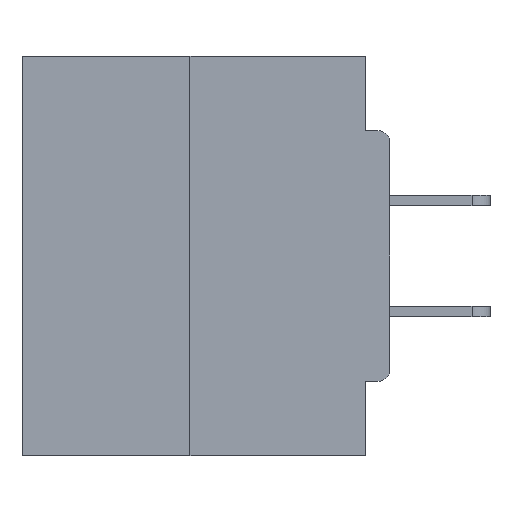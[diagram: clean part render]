
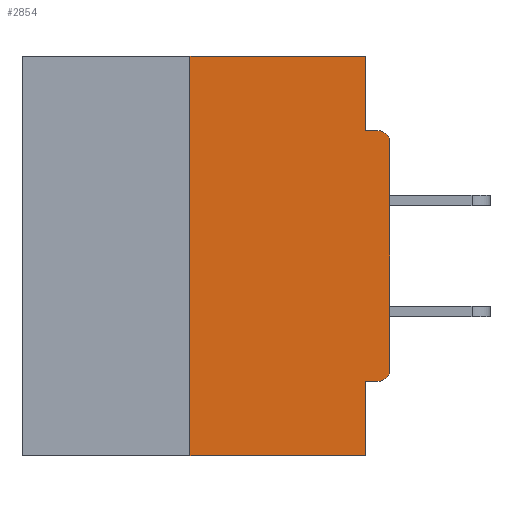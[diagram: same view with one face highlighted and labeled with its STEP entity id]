
A CAD part, left-side view. The second image highlights one B-rep face of the part: STEP entity #2854.
In plain terms, the highlighted planar face has unit normal (-1, 0, 0).
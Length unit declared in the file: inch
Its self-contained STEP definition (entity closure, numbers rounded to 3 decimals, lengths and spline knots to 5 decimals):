
#128 = CARTESIAN_POINT ( 'NONE',  ( 0., 0.25, 0. ) ) ;
#163 = LINE ( 'NONE', #9701, #3685 ) ;
#194 = LINE ( 'NONE', #17991, #10735 ) ;
#793 = EDGE_CURVE ( 'NONE', #3441, #19362, #4950, .T. ) ;
#2200 = VECTOR ( 'NONE', #20018, 39.37008 ) ;
#2360 = CARTESIAN_POINT ( 'NONE',  ( 0., 0.015, -0.0935 ) ) ;
#2854 = ADVANCED_FACE ( 'NONE', ( #17640 ), #22155, .F. ) ;
#3117 = CARTESIAN_POINT ( 'NONE',  ( 0., 0.031, -0.0935 ) ) ;
#3195 = AXIS2_PLACEMENT_3D ( 'NONE', #13177, #10878, #30624 ) ;
#3441 = VERTEX_POINT ( 'NONE', #32235 ) ;
#3685 = VECTOR ( 'NONE', #22270, 39.37008 ) ;
#4775 = LINE ( 'NONE', #26997, #11666 ) ;
#4950 = LINE ( 'NONE', #18474, #13860 ) ;
#4961 = ORIENTED_EDGE ( 'NONE', *, *, #5586, .T. ) ;
#5586 = EDGE_CURVE ( 'NONE', #31996, #8220, #15919, .T. ) ;
#6318 = VERTEX_POINT ( 'NONE', #6709 ) ;
#6709 = CARTESIAN_POINT ( 'NONE',  ( 0., 0.031, -0.4065 ) ) ;
#7233 = VECTOR ( 'NONE', #26794, 39.37008 ) ;
#7288 = VERTEX_POINT ( 'NONE', #28403 ) ;
#7358 = CARTESIAN_POINT ( 'NONE',  ( 0., 0., 0. ) ) ;
#8052 = DIRECTION ( 'NONE',  ( 0., -1., 0. ) ) ;
#8220 = VERTEX_POINT ( 'NONE', #25533 ) ;
#8669 = VECTOR ( 'NONE', #18846, 39.37008 ) ;
#9069 = LINE ( 'NONE', #18731, #8669 ) ;
#9150 = VERTEX_POINT ( 'NONE', #2360 ) ;
#9237 = ORIENTED_EDGE ( 'NONE', *, *, #793, .F. ) ;
#9400 = VERTEX_POINT ( 'NONE', #10531 ) ;
#9612 = ORIENTED_EDGE ( 'NONE', *, *, #17049, .F. ) ;
#9701 = CARTESIAN_POINT ( 'NONE',  ( 0., 0.46, -0.5 ) ) ;
#9727 = EDGE_CURVE ( 'NONE', #6318, #30747, #4775, .T. ) ;
#9931 = DIRECTION ( 'NONE',  ( 0., 0., -1. ) ) ;
#10371 = ORIENTED_EDGE ( 'NONE', *, *, #12258, .T. ) ;
#10531 = CARTESIAN_POINT ( 'NONE',  ( 0., 0., -0.1085 ) ) ;
#10735 = VECTOR ( 'NONE', #8052, 39.37008 ) ;
#10878 = DIRECTION ( 'NONE',  ( -1., 0., 0. ) ) ;
#11666 = VECTOR ( 'NONE', #17075, 39.37008 ) ;
#11903 = VERTEX_POINT ( 'NONE', #3117 ) ;
#12258 = EDGE_CURVE ( 'NONE', #8220, #9400, #12717, .T. ) ;
#12311 = CARTESIAN_POINT ( 'NONE',  ( 0., 0.015, -0.4065 ) ) ;
#12528 = CIRCLE ( 'NONE', #19348, 0.015 ) ;
#12717 = LINE ( 'NONE', #7358, #2200 ) ;
#12792 = EDGE_LOOP ( 'NONE', ( #9237, #24526, #14416, #16158, #17834, #4961, #10371, #30064, #14086, #9612 ) ) ;
#13177 = CARTESIAN_POINT ( 'NONE',  ( 0., 0.015, -0.3915 ) ) ;
#13860 = VECTOR ( 'NONE', #18144, 39.37008 ) ;
#13964 = EDGE_CURVE ( 'NONE', #7288, #3441, #30974, .T. ) ;
#14086 = ORIENTED_EDGE ( 'NONE', *, *, #20758, .F. ) ;
#14416 = ORIENTED_EDGE ( 'NONE', *, *, #23363, .T. ) ;
#14937 = DIRECTION ( 'NONE',  ( 1., 0., 0. ) ) ;
#15919 = CIRCLE ( 'NONE', #3195, 0.015 ) ;
#16158 = ORIENTED_EDGE ( 'NONE', *, *, #9727, .F. ) ;
#17049 = EDGE_CURVE ( 'NONE', #19362, #11903, #9069, .T. ) ;
#17075 = DIRECTION ( 'NONE',  ( 0., 0., -1. ) ) ;
#17348 = EDGE_CURVE ( 'NONE', #9400, #9150, #12528, .T. ) ;
#17640 = FACE_OUTER_BOUND ( 'NONE', #12792, .T. ) ;
#17834 = ORIENTED_EDGE ( 'NONE', *, *, #20898, .F. ) ;
#17991 = CARTESIAN_POINT ( 'NONE',  ( 0., 0., -0.0935 ) ) ;
#18144 = DIRECTION ( 'NONE',  ( 0., -1., 0. ) ) ;
#18474 = CARTESIAN_POINT ( 'NONE',  ( 0., 0.46, 0. ) ) ;
#18731 = CARTESIAN_POINT ( 'NONE',  ( 0., 0.031, 0. ) ) ;
#18846 = DIRECTION ( 'NONE',  ( 0., 0., -1. ) ) ;
#19348 = AXIS2_PLACEMENT_3D ( 'NONE', #22858, #22967, #27750 ) ;
#19362 = VERTEX_POINT ( 'NONE', #22046 ) ;
#19857 = CARTESIAN_POINT ( 'NONE',  ( 0., 0.46, 0. ) ) ;
#20018 = DIRECTION ( 'NONE',  ( 0., 0., 1. ) ) ;
#20758 = EDGE_CURVE ( 'NONE', #11903, #9150, #194, .T. ) ;
#20898 = EDGE_CURVE ( 'NONE', #31996, #6318, #30207, .T. ) ;
#21677 = CARTESIAN_POINT ( 'NONE',  ( 0., 0., -0.4065 ) ) ;
#22046 = CARTESIAN_POINT ( 'NONE',  ( 0., 0.031, 0. ) ) ;
#22155 = PLANE ( 'NONE',  #25495 ) ;
#22270 = DIRECTION ( 'NONE',  ( 0., -1., 0. ) ) ;
#22858 = CARTESIAN_POINT ( 'NONE',  ( 0., 0.015, -0.1085 ) ) ;
#22967 = DIRECTION ( 'NONE',  ( -1., 0., 0. ) ) ;
#23235 = VECTOR ( 'NONE', #29998, 39.37008 ) ;
#23363 = EDGE_CURVE ( 'NONE', #7288, #30747, #163, .T. ) ;
#24526 = ORIENTED_EDGE ( 'NONE', *, *, #13964, .F. ) ;
#25495 = AXIS2_PLACEMENT_3D ( 'NONE', #19857, #14937, #9931 ) ;
#25533 = CARTESIAN_POINT ( 'NONE',  ( 0., 0., -0.3915 ) ) ;
#26794 = DIRECTION ( 'NONE',  ( 0., 1., 0. ) ) ;
#26997 = CARTESIAN_POINT ( 'NONE',  ( 0., 0.031, -0.5 ) ) ;
#27750 = DIRECTION ( 'NONE',  ( 0., 0., -1. ) ) ;
#28403 = CARTESIAN_POINT ( 'NONE',  ( 0., 0.25, -0.5 ) ) ;
#29998 = DIRECTION ( 'NONE',  ( 0., 0., 1. ) ) ;
#30064 = ORIENTED_EDGE ( 'NONE', *, *, #17348, .T. ) ;
#30207 = LINE ( 'NONE', #21677, #7233 ) ;
#30572 = CARTESIAN_POINT ( 'NONE',  ( 0., 0.031, -0.5 ) ) ;
#30624 = DIRECTION ( 'NONE',  ( 0., 0., -1. ) ) ;
#30747 = VERTEX_POINT ( 'NONE', #30572 ) ;
#30974 = LINE ( 'NONE', #128, #23235 ) ;
#31996 = VERTEX_POINT ( 'NONE', #12311 ) ;
#32235 = CARTESIAN_POINT ( 'NONE',  ( 0., 0.25, 0. ) ) ;
